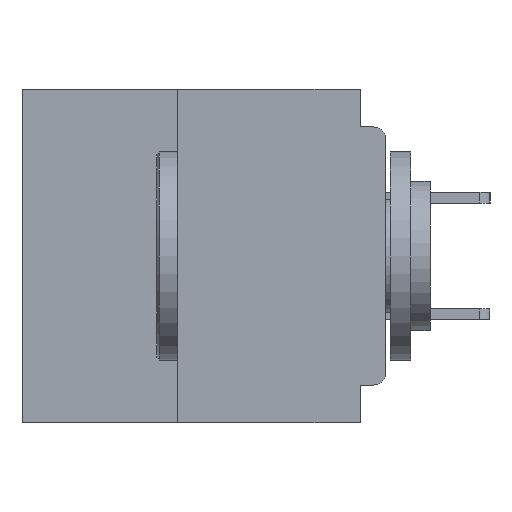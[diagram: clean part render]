
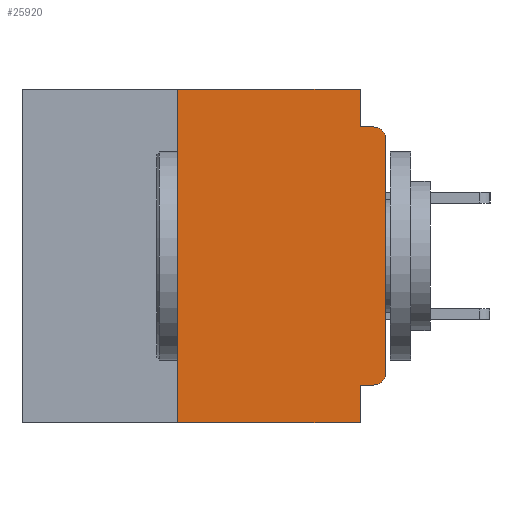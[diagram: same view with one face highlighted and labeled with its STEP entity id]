
A CAD part, left-side view. The second image highlights one B-rep face of the part: STEP entity #25920.
In plain terms, the highlighted planar face has unit normal (-1, 0, 0).
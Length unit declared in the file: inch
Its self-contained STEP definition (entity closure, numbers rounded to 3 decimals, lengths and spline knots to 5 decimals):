
#548 = DIRECTION ( 'NONE',  ( 0., 0., -1. ) ) ;
#798 = ORIENTED_EDGE ( 'NONE', *, *, #50235, .T. ) ;
#1142 = DIRECTION ( 'NONE',  ( 0., 0., -1. ) ) ;
#1873 = VERTEX_POINT ( 'NONE', #29847 ) ;
#1999 = ORIENTED_EDGE ( 'NONE', *, *, #28842, .T. ) ;
#4369 = CIRCLE ( 'NONE', #8137, 0.015 ) ;
#4697 = CARTESIAN_POINT ( 'NONE',  ( 0., 0.015, -0.34 ) ) ;
#5321 = CARTESIAN_POINT ( 'NONE',  ( 0., 0.437, 0. ) ) ;
#5750 = VERTEX_POINT ( 'NONE', #15141 ) ;
#7164 = VERTEX_POINT ( 'NONE', #46789 ) ;
#7193 = LINE ( 'NONE', #26605, #17445 ) ;
#8137 = AXIS2_PLACEMENT_3D ( 'NONE', #4697, #35105, #9073 ) ;
#8205 = LINE ( 'NONE', #20309, #29958 ) ;
#9073 = DIRECTION ( 'NONE',  ( 0., 0., -1. ) ) ;
#9700 = DIRECTION ( 'NONE',  ( 0., -1., 0. ) ) ;
#9840 = CARTESIAN_POINT ( 'NONE',  ( 0., 0.25, 0. ) ) ;
#10140 = VECTOR ( 'NONE', #51216, 39.37008 ) ;
#10478 = VECTOR ( 'NONE', #12709, 39.37008 ) ;
#10969 = ORIENTED_EDGE ( 'NONE', *, *, #30817, .F. ) ;
#11949 = ORIENTED_EDGE ( 'NONE', *, *, #44982, .F. ) ;
#12277 = EDGE_CURVE ( 'NONE', #7164, #29478, #4369, .T. ) ;
#12709 = DIRECTION ( 'NONE',  ( 0., -1., 0. ) ) ;
#12873 = ORIENTED_EDGE ( 'NONE', *, *, #24940, .F. ) ;
#13671 = ORIENTED_EDGE ( 'NONE', *, *, #17606, .F. ) ;
#14136 = PLANE ( 'NONE',  #24571 ) ;
#14589 = LINE ( 'NONE', #34528, #10478 ) ;
#15141 = CARTESIAN_POINT ( 'NONE',  ( 0., 0., -0.06 ) ) ;
#15730 = VECTOR ( 'NONE', #9700, 39.37008 ) ;
#17445 = VECTOR ( 'NONE', #35340, 39.37008 ) ;
#17606 = EDGE_CURVE ( 'NONE', #7164, #37047, #42138, .T. ) ;
#18063 = VERTEX_POINT ( 'NONE', #50014 ) ;
#18510 = DIRECTION ( 'NONE',  ( 1., 0., 0. ) ) ;
#20073 = CARTESIAN_POINT ( 'NONE',  ( 0., 0.25, -0.4 ) ) ;
#20309 = CARTESIAN_POINT ( 'NONE',  ( 0., 0.031, 0. ) ) ;
#20647 = ORIENTED_EDGE ( 'NONE', *, *, #12277, .T. ) ;
#21697 = LINE ( 'NONE', #25074, #10140 ) ;
#22036 = CARTESIAN_POINT ( 'NONE',  ( 0., 0.031, 0. ) ) ;
#24571 = AXIS2_PLACEMENT_3D ( 'NONE', #44535, #18510, #48841 ) ;
#24791 = CARTESIAN_POINT ( 'NONE',  ( 0., 0.015, -0.045 ) ) ;
#24940 = EDGE_CURVE ( 'NONE', #42667, #18063, #8205, .T. ) ;
#25074 = CARTESIAN_POINT ( 'NONE',  ( 0., 0.25, -0.4 ) ) ;
#25920 = ADVANCED_FACE ( 'NONE', ( #48853 ), #14136, .F. ) ;
#26605 = CARTESIAN_POINT ( 'NONE',  ( 0., 0., 0. ) ) ;
#27228 = DIRECTION ( 'NONE',  ( -1., 0., 0. ) ) ;
#27260 = ORIENTED_EDGE ( 'NONE', *, *, #40427, .T. ) ;
#28842 = EDGE_CURVE ( 'NONE', #55472, #1873, #14589, .T. ) ;
#29040 = DIRECTION ( 'NONE',  ( 0., 1., 0. ) ) ;
#29091 = ORIENTED_EDGE ( 'NONE', *, *, #32902, .F. ) ;
#29478 = VERTEX_POINT ( 'NONE', #29735 ) ;
#29735 = CARTESIAN_POINT ( 'NONE',  ( 0., 0., -0.34 ) ) ;
#29847 = CARTESIAN_POINT ( 'NONE',  ( 0., 0.031, -0.4 ) ) ;
#29958 = VECTOR ( 'NONE', #50633, 39.37008 ) ;
#30817 = EDGE_CURVE ( 'NONE', #37047, #1873, #54301, .T. ) ;
#31751 = LINE ( 'NONE', #55364, #52046 ) ;
#32902 = EDGE_CURVE ( 'NONE', #18063, #51800, #31751, .T. ) ;
#33378 = CARTESIAN_POINT ( 'NONE',  ( 0., 0., -0.355 ) ) ;
#33822 = DIRECTION ( 'NONE',  ( 0., -1., 0. ) ) ;
#34528 = CARTESIAN_POINT ( 'NONE',  ( 0., 0.437, -0.4 ) ) ;
#35105 = DIRECTION ( 'NONE',  ( -1., 0., 0. ) ) ;
#35340 = DIRECTION ( 'NONE',  ( 0., 0., 1. ) ) ;
#37047 = VERTEX_POINT ( 'NONE', #49596 ) ;
#37446 = LINE ( 'NONE', #5321, #15730 ) ;
#40427 = EDGE_CURVE ( 'NONE', #29478, #5750, #7193, .T. ) ;
#40783 = VECTOR ( 'NONE', #29040, 39.37008 ) ;
#42138 = LINE ( 'NONE', #33378, #40783 ) ;
#42667 = VERTEX_POINT ( 'NONE', #22036 ) ;
#42889 = VECTOR ( 'NONE', #548, 39.37008 ) ;
#43847 = ORIENTED_EDGE ( 'NONE', *, *, #49773, .F. ) ;
#44535 = CARTESIAN_POINT ( 'NONE',  ( 0., 0.437, 0. ) ) ;
#44982 = EDGE_CURVE ( 'NONE', #48090, #42667, #37446, .T. ) ;
#46789 = CARTESIAN_POINT ( 'NONE',  ( 0., 0.015, -0.355 ) ) ;
#48090 = VERTEX_POINT ( 'NONE', #9840 ) ;
#48280 = CARTESIAN_POINT ( 'NONE',  ( 0., 0.031, -0.4 ) ) ;
#48841 = DIRECTION ( 'NONE',  ( 0., 0., -1. ) ) ;
#48853 = FACE_OUTER_BOUND ( 'NONE', #54812, .T. ) ;
#49596 = CARTESIAN_POINT ( 'NONE',  ( 0., 0.031, -0.355 ) ) ;
#49773 = EDGE_CURVE ( 'NONE', #55472, #48090, #21697, .T. ) ;
#50014 = CARTESIAN_POINT ( 'NONE',  ( 0., 0.031, -0.045 ) ) ;
#50235 = EDGE_CURVE ( 'NONE', #5750, #51800, #53459, .T. ) ;
#50633 = DIRECTION ( 'NONE',  ( 0., 0., -1. ) ) ;
#51216 = DIRECTION ( 'NONE',  ( 0., 0., 1. ) ) ;
#51776 = AXIS2_PLACEMENT_3D ( 'NONE', #53139, #27228, #1142 ) ;
#51800 = VERTEX_POINT ( 'NONE', #24791 ) ;
#52046 = VECTOR ( 'NONE', #33822, 39.37008 ) ;
#53139 = CARTESIAN_POINT ( 'NONE',  ( 0., 0.015, -0.06 ) ) ;
#53459 = CIRCLE ( 'NONE', #51776, 0.015 ) ;
#54301 = LINE ( 'NONE', #48280, #42889 ) ;
#54812 = EDGE_LOOP ( 'NONE', ( #27260, #798, #29091, #12873, #11949, #43847, #1999, #10969, #13671, #20647 ) ) ;
#55364 = CARTESIAN_POINT ( 'NONE',  ( 0., 0., -0.045 ) ) ;
#55472 = VERTEX_POINT ( 'NONE', #20073 ) ;
